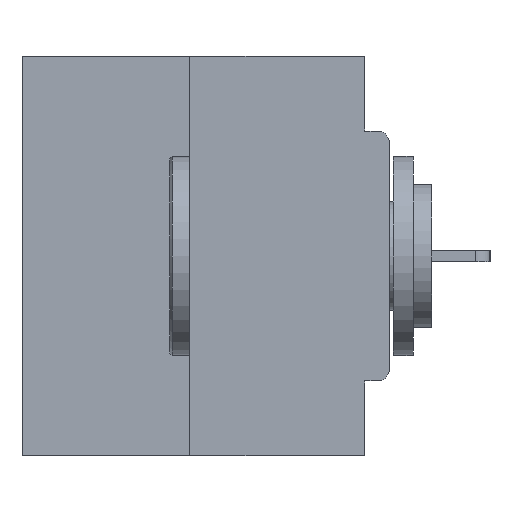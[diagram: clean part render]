
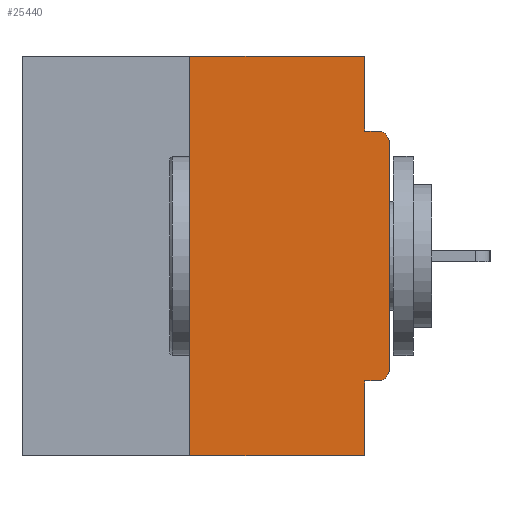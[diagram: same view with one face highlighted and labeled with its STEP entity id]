
A CAD part, left-side view. The second image highlights one B-rep face of the part: STEP entity #25440.
In plain terms, the highlighted planar face has unit normal (-1, 0, 0).
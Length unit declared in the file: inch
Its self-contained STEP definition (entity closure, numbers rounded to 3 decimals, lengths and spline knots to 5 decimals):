
#165 = DIRECTION ( 'NONE',  ( 0., 0., 1. ) ) ;
#441 = CARTESIAN_POINT ( 'NONE',  ( 0., 0.25, 0. ) ) ;
#610 = EDGE_CURVE ( 'NONE', #5273, #5819, #7512, .T. ) ;
#2788 = CARTESIAN_POINT ( 'NONE',  ( 0., 0., -0.0935 ) ) ;
#2911 = DIRECTION ( 'NONE',  ( 0., -1., 0. ) ) ;
#3150 = FACE_OUTER_BOUND ( 'NONE', #23077, .T. ) ;
#3156 = DIRECTION ( 'NONE',  ( 0., -1., 0. ) ) ;
#4179 = ORIENTED_EDGE ( 'NONE', *, *, #12132, .F. ) ;
#4580 = VECTOR ( 'NONE', #8593, 39.37008 ) ;
#4895 = VECTOR ( 'NONE', #21799, 39.37008 ) ;
#5273 = VERTEX_POINT ( 'NONE', #15289 ) ;
#5764 = CARTESIAN_POINT ( 'NONE',  ( 0., 0.015, -0.0935 ) ) ;
#5819 = VERTEX_POINT ( 'NONE', #6542 ) ;
#5950 = VECTOR ( 'NONE', #20150, 39.37008 ) ;
#6292 = LINE ( 'NONE', #8635, #4895 ) ;
#6542 = CARTESIAN_POINT ( 'NONE',  ( 0., 0.031, -0.5 ) ) ;
#6971 = LINE ( 'NONE', #11513, #5950 ) ;
#7191 = DIRECTION ( 'NONE',  ( 0., -1., 0. ) ) ;
#7512 = LINE ( 'NONE', #9572, #9237 ) ;
#7598 = VECTOR ( 'NONE', #165, 39.37008 ) ;
#7612 = VERTEX_POINT ( 'NONE', #21216 ) ;
#7835 = ORIENTED_EDGE ( 'NONE', *, *, #610, .F. ) ;
#8248 = EDGE_CURVE ( 'NONE', #27108, #27463, #19443, .T. ) ;
#8302 = CARTESIAN_POINT ( 'NONE',  ( 0., 0.031, 0. ) ) ;
#8593 = DIRECTION ( 'NONE',  ( 0., 0., -1. ) ) ;
#8635 = CARTESIAN_POINT ( 'NONE',  ( 0., 0., -0.4065 ) ) ;
#8662 = CIRCLE ( 'NONE', #15227, 0.015 ) ;
#9085 = CARTESIAN_POINT ( 'NONE',  ( 0., 0.015, -0.3915 ) ) ;
#9237 = VECTOR ( 'NONE', #18521, 39.37008 ) ;
#9572 = CARTESIAN_POINT ( 'NONE',  ( 0., 0.031, -0.5 ) ) ;
#9896 = PLANE ( 'NONE',  #20077 ) ;
#9946 = CARTESIAN_POINT ( 'NONE',  ( 0., 0.46, 0. ) ) ;
#10151 = CARTESIAN_POINT ( 'NONE',  ( 0., 0.031, 0. ) ) ;
#10336 = VECTOR ( 'NONE', #7191, 39.37008 ) ;
#10503 = VERTEX_POINT ( 'NONE', #22267 ) ;
#11013 = ORIENTED_EDGE ( 'NONE', *, *, #21162, .T. ) ;
#11338 = ORIENTED_EDGE ( 'NONE', *, *, #8248, .F. ) ;
#11513 = CARTESIAN_POINT ( 'NONE',  ( 0., 0., 0. ) ) ;
#11672 = DIRECTION ( 'NONE',  ( 0., 0., -1. ) ) ;
#11983 = CIRCLE ( 'NONE', #21790, 0.015 ) ;
#12132 = EDGE_CURVE ( 'NONE', #19422, #16986, #20651, .T. ) ;
#14494 = LINE ( 'NONE', #9946, #19453 ) ;
#14722 = VECTOR ( 'NONE', #3156, 39.37008 ) ;
#14752 = CARTESIAN_POINT ( 'NONE',  ( 0., 0.25, 0. ) ) ;
#15227 = AXIS2_PLACEMENT_3D ( 'NONE', #9085, #22825, #18038 ) ;
#15289 = CARTESIAN_POINT ( 'NONE',  ( 0., 0.031, -0.4065 ) ) ;
#15548 = EDGE_CURVE ( 'NONE', #19422, #5819, #25423, .T. ) ;
#15613 = DIRECTION ( 'NONE',  ( -1., 0., 0. ) ) ;
#16023 = CARTESIAN_POINT ( 'NONE',  ( 0., 0.015, -0.1085 ) ) ;
#16032 = ORIENTED_EDGE ( 'NONE', *, *, #22091, .T. ) ;
#16359 = EDGE_CURVE ( 'NONE', #16986, #27108, #14494, .T. ) ;
#16859 = ORIENTED_EDGE ( 'NONE', *, *, #16359, .F. ) ;
#16986 = VERTEX_POINT ( 'NONE', #14752 ) ;
#17255 = ORIENTED_EDGE ( 'NONE', *, *, #18075, .T. ) ;
#18038 = DIRECTION ( 'NONE',  ( 0., 0., -1. ) ) ;
#18075 = EDGE_CURVE ( 'NONE', #7612, #18819, #8662, .T. ) ;
#18343 = CARTESIAN_POINT ( 'NONE',  ( 0., 0.031, -0.0935 ) ) ;
#18415 = CARTESIAN_POINT ( 'NONE',  ( 0., 0.46, -0.5 ) ) ;
#18521 = DIRECTION ( 'NONE',  ( 0., 0., -1. ) ) ;
#18819 = VERTEX_POINT ( 'NONE', #25766 ) ;
#19422 = VERTEX_POINT ( 'NONE', #22186 ) ;
#19443 = LINE ( 'NONE', #8302, #4580 ) ;
#19453 = VECTOR ( 'NONE', #2911, 39.37008 ) ;
#20077 = AXIS2_PLACEMENT_3D ( 'NONE', #20728, #21008, #11672 ) ;
#20146 = EDGE_CURVE ( 'NONE', #7612, #5273, #6292, .T. ) ;
#20150 = DIRECTION ( 'NONE',  ( 0., 0., 1. ) ) ;
#20651 = LINE ( 'NONE', #441, #7598 ) ;
#20728 = CARTESIAN_POINT ( 'NONE',  ( 0., 0.46, 0. ) ) ;
#21008 = DIRECTION ( 'NONE',  ( 1., 0., 0. ) ) ;
#21052 = VERTEX_POINT ( 'NONE', #5764 ) ;
#21162 = EDGE_CURVE ( 'NONE', #10503, #21052, #11983, .T. ) ;
#21216 = CARTESIAN_POINT ( 'NONE',  ( 0., 0.015, -0.4065 ) ) ;
#21744 = ORIENTED_EDGE ( 'NONE', *, *, #15548, .T. ) ;
#21790 = AXIS2_PLACEMENT_3D ( 'NONE', #16023, #15613, #22433 ) ;
#21799 = DIRECTION ( 'NONE',  ( 0., 1., 0. ) ) ;
#22091 = EDGE_CURVE ( 'NONE', #18819, #10503, #6971, .T. ) ;
#22186 = CARTESIAN_POINT ( 'NONE',  ( 0., 0.25, -0.5 ) ) ;
#22267 = CARTESIAN_POINT ( 'NONE',  ( 0., 0., -0.1085 ) ) ;
#22433 = DIRECTION ( 'NONE',  ( 0., 0., -1. ) ) ;
#22744 = ORIENTED_EDGE ( 'NONE', *, *, #27470, .F. ) ;
#22825 = DIRECTION ( 'NONE',  ( -1., 0., 0. ) ) ;
#23077 = EDGE_LOOP ( 'NONE', ( #16859, #4179, #21744, #7835, #23223, #17255, #16032, #11013, #22744, #11338 ) ) ;
#23223 = ORIENTED_EDGE ( 'NONE', *, *, #20146, .F. ) ;
#25047 = LINE ( 'NONE', #2788, #10336 ) ;
#25423 = LINE ( 'NONE', #18415, #14722 ) ;
#25440 = ADVANCED_FACE ( 'NONE', ( #3150 ), #9896, .F. ) ;
#25766 = CARTESIAN_POINT ( 'NONE',  ( 0., 0., -0.3915 ) ) ;
#27108 = VERTEX_POINT ( 'NONE', #10151 ) ;
#27463 = VERTEX_POINT ( 'NONE', #18343 ) ;
#27470 = EDGE_CURVE ( 'NONE', #27463, #21052, #25047, .T. ) ;
